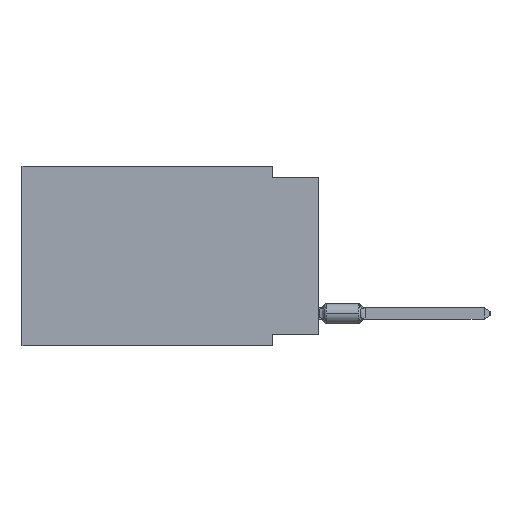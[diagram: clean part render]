
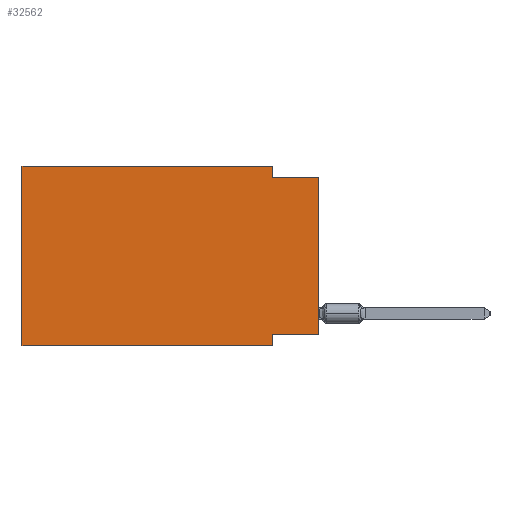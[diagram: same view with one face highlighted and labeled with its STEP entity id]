
A CAD part, left-side view. The second image highlights one B-rep face of the part: STEP entity #32562.
In plain terms, the highlighted planar face has unit normal (-1, 0, 0).
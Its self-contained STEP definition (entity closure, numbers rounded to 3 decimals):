
#250 = VECTOR ( 'NONE', #57971, 1000. ) ;
#1627 = EDGE_CURVE ( 'NONE', #47249, #14406, #5578, .T. ) ;
#3185 = VECTOR ( 'NONE', #43796, 1000. ) ;
#3407 = VERTEX_POINT ( 'NONE', #39294 ) ;
#4435 = EDGE_LOOP ( 'NONE', ( #8630, #54750, #20891, #5521, #53446, #67383, #38316, #20442 ) ) ;
#4992 = VERTEX_POINT ( 'NONE', #63980 ) ;
#5521 = ORIENTED_EDGE ( 'NONE', *, *, #5966, .F. ) ;
#5578 = LINE ( 'NONE', #11366, #69748 ) ;
#5792 = LINE ( 'NONE', #43864, #42170 ) ;
#5947 = DIRECTION ( 'NONE',  ( 0., 0., -1. ) ) ;
#5966 = EDGE_CURVE ( 'NONE', #57810, #47249, #22494, .T. ) ;
#8630 = ORIENTED_EDGE ( 'NONE', *, *, #11801, .T. ) ;
#9811 = LINE ( 'NONE', #31943, #31227 ) ;
#9870 = CARTESIAN_POINT ( 'NONE',  ( 0., 2.54, -9.906 ) ) ;
#10150 = CARTESIAN_POINT ( 'NONE',  ( 0., 2.54, -0.635 ) ) ;
#10210 = LINE ( 'NONE', #9870, #37299 ) ;
#11366 = CARTESIAN_POINT ( 'NONE',  ( 0., 2.54, 0. ) ) ;
#11801 = EDGE_CURVE ( 'NONE', #46924, #31843, #9811, .T. ) ;
#14406 = VERTEX_POINT ( 'NONE', #10150 ) ;
#18313 = EDGE_CURVE ( 'NONE', #3407, #56768, #59918, .T. ) ;
#20442 = ORIENTED_EDGE ( 'NONE', *, *, #68130, .F. ) ;
#20891 = ORIENTED_EDGE ( 'NONE', *, *, #1627, .F. ) ;
#21811 = DIRECTION ( 'NONE',  ( 0., -1., 0. ) ) ;
#22494 = LINE ( 'NONE', #28317, #63249 ) ;
#24792 = CARTESIAN_POINT ( 'NONE',  ( 0., 0., -9.271 ) ) ;
#25356 = CARTESIAN_POINT ( 'NONE',  ( 0., 16.383, 0. ) ) ;
#27143 = CARTESIAN_POINT ( 'NONE',  ( 0., 16.383, 0. ) ) ;
#28317 = CARTESIAN_POINT ( 'NONE',  ( 0., 16.383, 0. ) ) ;
#29502 = CARTESIAN_POINT ( 'NONE',  ( 0., 16.383, 0. ) ) ;
#31227 = VECTOR ( 'NONE', #32298, 1000. ) ;
#31843 = VERTEX_POINT ( 'NONE', #57499 ) ;
#31943 = CARTESIAN_POINT ( 'NONE',  ( 0., 0., 0. ) ) ;
#32298 = DIRECTION ( 'NONE',  ( 0., 0., 1. ) ) ;
#32562 = ADVANCED_FACE ( 'NONE', ( #46158 ), #57051, .F. ) ;
#33558 = EDGE_CURVE ( 'NONE', #4992, #56768, #10210, .T. ) ;
#37299 = VECTOR ( 'NONE', #49736, 1000. ) ;
#37816 = VECTOR ( 'NONE', #21811, 1000. ) ;
#38316 = ORIENTED_EDGE ( 'NONE', *, *, #33558, .F. ) ;
#38943 = DIRECTION ( 'NONE',  ( 0., 0., -1. ) ) ;
#39294 = CARTESIAN_POINT ( 'NONE',  ( 0., 16.383, -9.906 ) ) ;
#42170 = VECTOR ( 'NONE', #60544, 1000. ) ;
#43796 = DIRECTION ( 'NONE',  ( 0., 0., 1. ) ) ;
#43864 = CARTESIAN_POINT ( 'NONE',  ( 0., 0., -0.635 ) ) ;
#44710 = EDGE_CURVE ( 'NONE', #3407, #57810, #64468, .T. ) ;
#45379 = CARTESIAN_POINT ( 'NONE',  ( 0., 2.54, 0. ) ) ;
#46158 = FACE_OUTER_BOUND ( 'NONE', #4435, .T. ) ;
#46924 = VERTEX_POINT ( 'NONE', #24792 ) ;
#47249 = VERTEX_POINT ( 'NONE', #45379 ) ;
#49736 = DIRECTION ( 'NONE',  ( 0., 0., -1. ) ) ;
#51611 = DIRECTION ( 'NONE',  ( 1., 0., 0. ) ) ;
#53446 = ORIENTED_EDGE ( 'NONE', *, *, #44710, .F. ) ;
#54470 = AXIS2_PLACEMENT_3D ( 'NONE', #29502, #51611, #38943 ) ;
#54572 = LINE ( 'NONE', #63739, #250 ) ;
#54750 = ORIENTED_EDGE ( 'NONE', *, *, #69243, .F. ) ;
#55489 = DIRECTION ( 'NONE',  ( 0., -1., 0. ) ) ;
#56768 = VERTEX_POINT ( 'NONE', #70958 ) ;
#57051 = PLANE ( 'NONE',  #54470 ) ;
#57499 = CARTESIAN_POINT ( 'NONE',  ( 0., 0., -0.635 ) ) ;
#57810 = VERTEX_POINT ( 'NONE', #25356 ) ;
#57971 = DIRECTION ( 'NONE',  ( 0., 1., 0. ) ) ;
#59918 = LINE ( 'NONE', #71126, #37816 ) ;
#60544 = DIRECTION ( 'NONE',  ( 0., -1., 0. ) ) ;
#63249 = VECTOR ( 'NONE', #55489, 1000. ) ;
#63739 = CARTESIAN_POINT ( 'NONE',  ( 0., 0., -9.271 ) ) ;
#63980 = CARTESIAN_POINT ( 'NONE',  ( 0., 2.54, -9.271 ) ) ;
#64468 = LINE ( 'NONE', #27143, #3185 ) ;
#67383 = ORIENTED_EDGE ( 'NONE', *, *, #18313, .T. ) ;
#68130 = EDGE_CURVE ( 'NONE', #46924, #4992, #54572, .T. ) ;
#69243 = EDGE_CURVE ( 'NONE', #14406, #31843, #5792, .T. ) ;
#69748 = VECTOR ( 'NONE', #5947, 1000. ) ;
#70958 = CARTESIAN_POINT ( 'NONE',  ( 0., 2.54, -9.906 ) ) ;
#71126 = CARTESIAN_POINT ( 'NONE',  ( 0., 16.383, -9.906 ) ) ;
